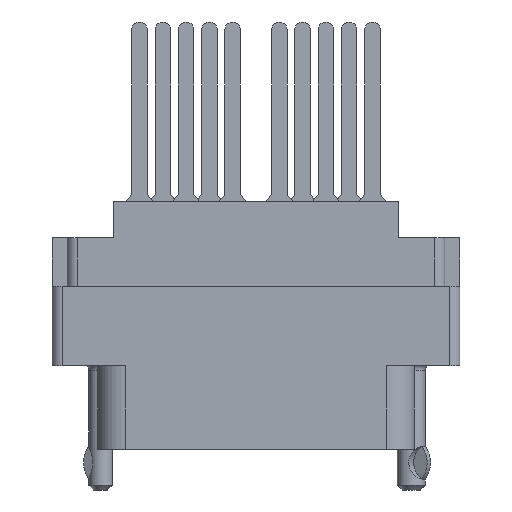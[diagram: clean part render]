
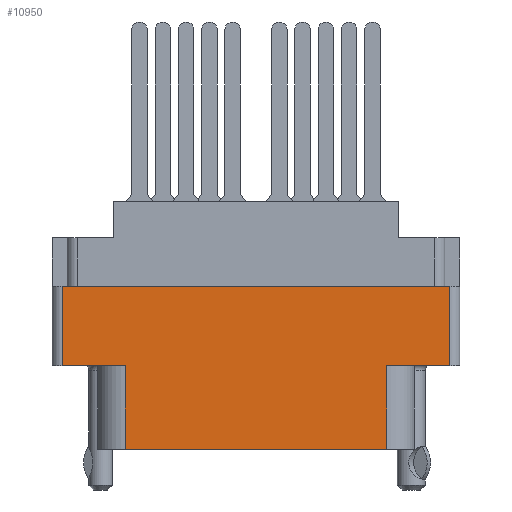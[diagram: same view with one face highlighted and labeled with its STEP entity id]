
A CAD part, front view. The second image highlights one B-rep face of the part: STEP entity #10950.
In plain terms, the highlighted planar face has unit normal (0, -1, 0).
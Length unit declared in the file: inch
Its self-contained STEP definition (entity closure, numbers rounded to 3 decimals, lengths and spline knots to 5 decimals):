
#3 = DIRECTION ( 'NONE',  ( -1., 0., 0. ) ) ;
#123 = VERTEX_POINT ( 'NONE', #27472 ) ;
#1155 = VECTOR ( 'NONE', #24030, 39.37008 ) ;
#2525 = DIRECTION ( 'NONE',  ( 0., 0., 1. ) ) ;
#2627 = VERTEX_POINT ( 'NONE', #19411 ) ;
#2959 = LINE ( 'NONE', #37349, #21644 ) ;
#3809 = VERTEX_POINT ( 'NONE', #36119 ) ;
#4090 = DIRECTION ( 'NONE',  ( 0., 0., -1. ) ) ;
#4806 = CARTESIAN_POINT ( 'NONE',  ( -0.42052, -0.343, -0.529 ) ) ;
#4868 = VECTOR ( 'NONE', #13655, 39.37008 ) ;
#5817 = ORIENTED_EDGE ( 'NONE', *, *, #23288, .T. ) ;
#6519 = LINE ( 'NONE', #22422, #21099 ) ;
#7284 = CARTESIAN_POINT ( 'NONE',  ( -0.42052, -0.343, -0.798 ) ) ;
#7397 = VECTOR ( 'NONE', #4090, 39.37008 ) ;
#8413 = LINE ( 'NONE', #30658, #18868 ) ;
#8480 = EDGE_LOOP ( 'NONE', ( #17783, #5817, #29208, #14810, #14042, #21524, #27521, #11641 ) ) ;
#8689 = VERTEX_POINT ( 'NONE', #4806 ) ;
#8967 = DIRECTION ( 'NONE',  ( 1., 0., 0. ) ) ;
#9439 = CARTESIAN_POINT ( 'NONE',  ( 0.624, -0.343, -0.798 ) ) ;
#9673 = AXIS2_PLACEMENT_3D ( 'NONE', #31829, #12070, #20471 ) ;
#10599 = EDGE_CURVE ( 'NONE', #17446, #30019, #27529, .T. ) ;
#10950 = ADVANCED_FACE ( 'NONE', ( #32900 ), #14873, .T. ) ;
#11215 = EDGE_CURVE ( 'NONE', #17446, #34308, #2959, .T. ) ;
#11641 = ORIENTED_EDGE ( 'NONE', *, *, #10599, .T. ) ;
#12070 = DIRECTION ( 'NONE',  ( 0., -1., 0. ) ) ;
#12840 = DIRECTION ( 'NONE',  ( 1., 0., 0. ) ) ;
#13565 = LINE ( 'NONE', #13919, #4868 ) ;
#13655 = DIRECTION ( 'NONE',  ( 1., 0., 0. ) ) ;
#13919 = CARTESIAN_POINT ( 'NONE',  ( 0., -0.343, -0.529 ) ) ;
#14042 = ORIENTED_EDGE ( 'NONE', *, *, #17707, .T. ) ;
#14810 = ORIENTED_EDGE ( 'NONE', *, *, #18204, .T. ) ;
#14873 = PLANE ( 'NONE',  #9673 ) ;
#16251 = VECTOR ( 'NONE', #8967, 39.37008 ) ;
#17184 = LINE ( 'NONE', #23031, #35711 ) ;
#17446 = VERTEX_POINT ( 'NONE', #25322 ) ;
#17707 = EDGE_CURVE ( 'NONE', #32791, #3809, #6519, .T. ) ;
#17783 = ORIENTED_EDGE ( 'NONE', *, *, #19475, .F. ) ;
#18204 = EDGE_CURVE ( 'NONE', #8689, #32791, #31018, .T. ) ;
#18868 = VECTOR ( 'NONE', #22212, 39.37008 ) ;
#19411 = CARTESIAN_POINT ( 'NONE',  ( -0.624, -0.343, -0.529 ) ) ;
#19475 = EDGE_CURVE ( 'NONE', #123, #30019, #23520, .T. ) ;
#20471 = DIRECTION ( 'NONE',  ( 0., 0., -1. ) ) ;
#21018 = EDGE_CURVE ( 'NONE', #2627, #8689, #13565, .T. ) ;
#21099 = VECTOR ( 'NONE', #12840, 39.37008 ) ;
#21187 = EDGE_CURVE ( 'NONE', #3809, #34308, #17184, .T. ) ;
#21524 = ORIENTED_EDGE ( 'NONE', *, *, #21187, .T. ) ;
#21644 = VECTOR ( 'NONE', #3, 39.37008 ) ;
#22212 = DIRECTION ( 'NONE',  ( 0., 0., -1. ) ) ;
#22422 = CARTESIAN_POINT ( 'NONE',  ( -0.656, -0.343, -0.798 ) ) ;
#23031 = CARTESIAN_POINT ( 'NONE',  ( 0.42052, -0.343, -0.529 ) ) ;
#23288 = EDGE_CURVE ( 'NONE', #123, #2627, #8413, .T. ) ;
#23520 = LINE ( 'NONE', #25859, #16251 ) ;
#24030 = DIRECTION ( 'NONE',  ( 0., 0., 1. ) ) ;
#24354 = CARTESIAN_POINT ( 'NONE',  ( -0.42052, -0.343, -0.798 ) ) ;
#24843 = CARTESIAN_POINT ( 'NONE',  ( 0.42052, -0.343, -0.529 ) ) ;
#25322 = CARTESIAN_POINT ( 'NONE',  ( 0.624, -0.343, -0.529 ) ) ;
#25859 = CARTESIAN_POINT ( 'NONE',  ( 0., -0.343, -0.274 ) ) ;
#27472 = CARTESIAN_POINT ( 'NONE',  ( -0.624, -0.343, -0.274 ) ) ;
#27521 = ORIENTED_EDGE ( 'NONE', *, *, #11215, .F. ) ;
#27529 = LINE ( 'NONE', #9439, #1155 ) ;
#29208 = ORIENTED_EDGE ( 'NONE', *, *, #21018, .T. ) ;
#30019 = VERTEX_POINT ( 'NONE', #35098 ) ;
#30658 = CARTESIAN_POINT ( 'NONE',  ( -0.624, -0.343, -0.798 ) ) ;
#31018 = LINE ( 'NONE', #7284, #7397 ) ;
#31829 = CARTESIAN_POINT ( 'NONE',  ( -0.656, -0.343, -0.798 ) ) ;
#32791 = VERTEX_POINT ( 'NONE', #24354 ) ;
#32900 = FACE_OUTER_BOUND ( 'NONE', #8480, .T. ) ;
#34308 = VERTEX_POINT ( 'NONE', #24843 ) ;
#35098 = CARTESIAN_POINT ( 'NONE',  ( 0.624, -0.343, -0.274 ) ) ;
#35711 = VECTOR ( 'NONE', #2525, 39.37008 ) ;
#36119 = CARTESIAN_POINT ( 'NONE',  ( 0.42052, -0.343, -0.798 ) ) ;
#37349 = CARTESIAN_POINT ( 'NONE',  ( 0., -0.343, -0.529 ) ) ;
